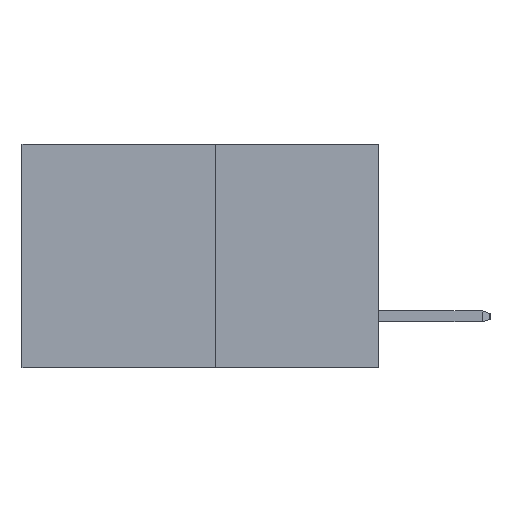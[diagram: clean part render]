
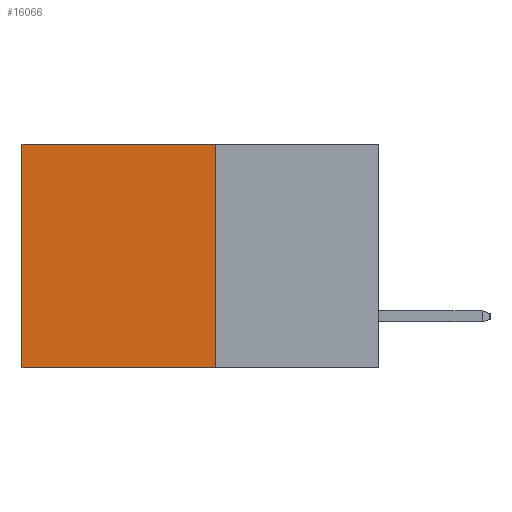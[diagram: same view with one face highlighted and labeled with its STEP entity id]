
A CAD part, left-side view. The second image highlights one B-rep face of the part: STEP entity #16066.
In plain terms, the highlighted planar face has unit normal (-1, 0, 0).
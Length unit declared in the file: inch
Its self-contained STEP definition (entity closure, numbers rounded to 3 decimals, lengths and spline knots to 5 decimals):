
#48 = CARTESIAN_POINT ( 'NONE',  ( 0.277, 0.59, 0. ) ) ;
#314 = PLANE ( 'NONE',  #7828 ) ;
#431 = ORIENTED_EDGE ( 'NONE', *, *, #12556, .T. ) ;
#1058 = EDGE_LOOP ( 'NONE', ( #3454, #16050, #4672, #431 ) ) ;
#1329 = VERTEX_POINT ( 'NONE', #2291 ) ;
#2291 = CARTESIAN_POINT ( 'NONE',  ( 0.277, 0.27, 0. ) ) ;
#3287 = VERTEX_POINT ( 'NONE', #16645 ) ;
#3454 = ORIENTED_EDGE ( 'NONE', *, *, #10769, .T. ) ;
#3532 = VECTOR ( 'NONE', #14666, 39.37008 ) ;
#3854 = CARTESIAN_POINT ( 'NONE',  ( 0.277, 0.27, -0.37 ) ) ;
#4380 = VERTEX_POINT ( 'NONE', #15212 ) ;
#4384 = VECTOR ( 'NONE', #18340, 39.37008 ) ;
#4672 = ORIENTED_EDGE ( 'NONE', *, *, #5148, .F. ) ;
#4909 = LINE ( 'NONE', #10092, #16643 ) ;
#5061 = DIRECTION ( 'NONE',  ( 1., 0., 0. ) ) ;
#5148 = EDGE_CURVE ( 'NONE', #1329, #3287, #16614, .T. ) ;
#7006 = DIRECTION ( 'NONE',  ( 0., 1., 0. ) ) ;
#7075 = CARTESIAN_POINT ( 'NONE',  ( 0.277, 0.59, -0.37 ) ) ;
#7828 = AXIS2_PLACEMENT_3D ( 'NONE', #11160, #5061, #15755 ) ;
#9823 = FACE_OUTER_BOUND ( 'NONE', #1058, .T. ) ;
#10092 = CARTESIAN_POINT ( 'NONE',  ( 0.277, 0.27, 0. ) ) ;
#10769 = EDGE_CURVE ( 'NONE', #16810, #4380, #11222, .T. ) ;
#11160 = CARTESIAN_POINT ( 'NONE',  ( 0.277, 0.27, -0.37 ) ) ;
#11222 = LINE ( 'NONE', #7075, #3532 ) ;
#11496 = DIRECTION ( 'NONE',  ( 0., 1., 0. ) ) ;
#12556 = EDGE_CURVE ( 'NONE', #1329, #16810, #4909, .T. ) ;
#13878 = LINE ( 'NONE', #3854, #17495 ) ;
#14666 = DIRECTION ( 'NONE',  ( 0., 0., -1. ) ) ;
#15212 = CARTESIAN_POINT ( 'NONE',  ( 0.277, 0.59, -0.37 ) ) ;
#15641 = EDGE_CURVE ( 'NONE', #3287, #4380, #13878, .T. ) ;
#15755 = DIRECTION ( 'NONE',  ( 0., 0., -1. ) ) ;
#16050 = ORIENTED_EDGE ( 'NONE', *, *, #15641, .F. ) ;
#16066 = ADVANCED_FACE ( 'NONE', ( #9823 ), #314, .F. ) ;
#16614 = LINE ( 'NONE', #18305, #4384 ) ;
#16643 = VECTOR ( 'NONE', #7006, 39.37008 ) ;
#16645 = CARTESIAN_POINT ( 'NONE',  ( 0.277, 0.27, -0.37 ) ) ;
#16810 = VERTEX_POINT ( 'NONE', #48 ) ;
#17495 = VECTOR ( 'NONE', #11496, 39.37008 ) ;
#18305 = CARTESIAN_POINT ( 'NONE',  ( 0.277, 0.27, -0.37 ) ) ;
#18340 = DIRECTION ( 'NONE',  ( 0., 0., -1. ) ) ;
